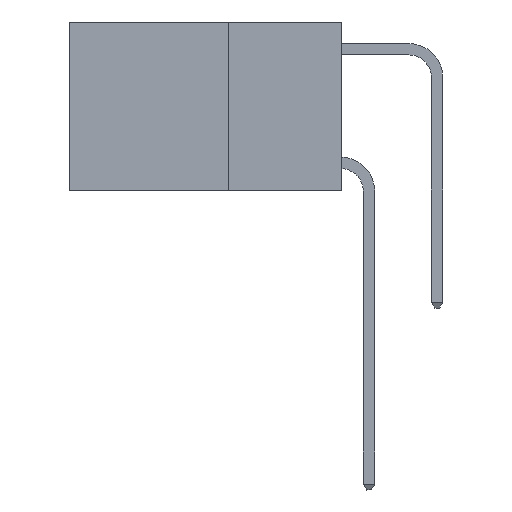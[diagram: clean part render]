
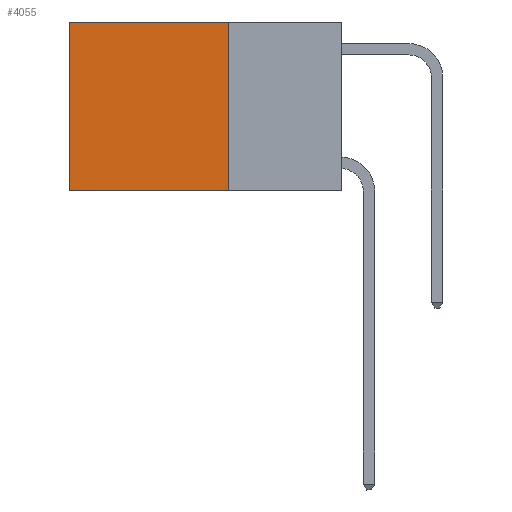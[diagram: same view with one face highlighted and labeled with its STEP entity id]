
A CAD part, left-side view. The second image highlights one B-rep face of the part: STEP entity #4055.
In plain terms, the highlighted planar face has unit normal (-1, 0, 0).
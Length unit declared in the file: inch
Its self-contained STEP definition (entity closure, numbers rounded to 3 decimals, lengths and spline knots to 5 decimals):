
#620 = LINE ( 'NONE', #3573, #11640 ) ;
#771 = DIRECTION ( 'NONE',  ( 0., 1., 0. ) ) ;
#1404 = EDGE_CURVE ( 'NONE', #15216, #15157, #620, .T. ) ;
#1546 = DIRECTION ( 'NONE',  ( 1., 0., 0. ) ) ;
#2364 = ORIENTED_EDGE ( 'NONE', *, *, #1404, .F. ) ;
#2609 = DIRECTION ( 'NONE',  ( 0., 0., -1. ) ) ;
#3573 = CARTESIAN_POINT ( 'NONE',  ( 0.2625, 0.25, -0.37 ) ) ;
#4014 = AXIS2_PLACEMENT_3D ( 'NONE', #6206, #1546, #2609 ) ;
#4055 = ADVANCED_FACE ( 'NONE', ( #6596 ), #8822, .F. ) ;
#4069 = EDGE_CURVE ( 'NONE', #10140, #15216, #9455, .T. ) ;
#5476 = CARTESIAN_POINT ( 'NONE',  ( 0.2625, 0.6, 0. ) ) ;
#5745 = VECTOR ( 'NONE', #10334, 39.37008 ) ;
#6206 = CARTESIAN_POINT ( 'NONE',  ( 0.2625, 0.25, 0. ) ) ;
#6596 = FACE_OUTER_BOUND ( 'NONE', #7143, .T. ) ;
#6911 = CARTESIAN_POINT ( 'NONE',  ( 0.2625, 0.6, -0.37 ) ) ;
#7143 = EDGE_LOOP ( 'NONE', ( #14193, #2364, #8917, #13430 ) ) ;
#8200 = CARTESIAN_POINT ( 'NONE',  ( 0.2625, 0.25, 0. ) ) ;
#8822 = PLANE ( 'NONE',  #4014 ) ;
#8917 = ORIENTED_EDGE ( 'NONE', *, *, #4069, .F. ) ;
#8978 = VECTOR ( 'NONE', #771, 39.37008 ) ;
#9415 = CARTESIAN_POINT ( 'NONE',  ( 0.2625, 0.6, 0. ) ) ;
#9455 = LINE ( 'NONE', #11212, #10226 ) ;
#10140 = VERTEX_POINT ( 'NONE', #12152 ) ;
#10226 = VECTOR ( 'NONE', #13664, 39.37008 ) ;
#10334 = DIRECTION ( 'NONE',  ( 0., 0., -1. ) ) ;
#10562 = VERTEX_POINT ( 'NONE', #9415 ) ;
#10751 = CARTESIAN_POINT ( 'NONE',  ( 0.2625, 0.25, -0.37 ) ) ;
#11212 = CARTESIAN_POINT ( 'NONE',  ( 0.2625, 0.25, 0. ) ) ;
#11640 = VECTOR ( 'NONE', #14531, 39.37008 ) ;
#12152 = CARTESIAN_POINT ( 'NONE',  ( 0.2625, 0.25, 0. ) ) ;
#13430 = ORIENTED_EDGE ( 'NONE', *, *, #15037, .T. ) ;
#13664 = DIRECTION ( 'NONE',  ( 0., 0., -1. ) ) ;
#14193 = ORIENTED_EDGE ( 'NONE', *, *, #14948, .T. ) ;
#14531 = DIRECTION ( 'NONE',  ( 0., 1., 0. ) ) ;
#14948 = EDGE_CURVE ( 'NONE', #10562, #15157, #15483, .T. ) ;
#15037 = EDGE_CURVE ( 'NONE', #10140, #10562, #15646, .T. ) ;
#15157 = VERTEX_POINT ( 'NONE', #6911 ) ;
#15216 = VERTEX_POINT ( 'NONE', #10751 ) ;
#15483 = LINE ( 'NONE', #5476, #5745 ) ;
#15646 = LINE ( 'NONE', #8200, #8978 ) ;
